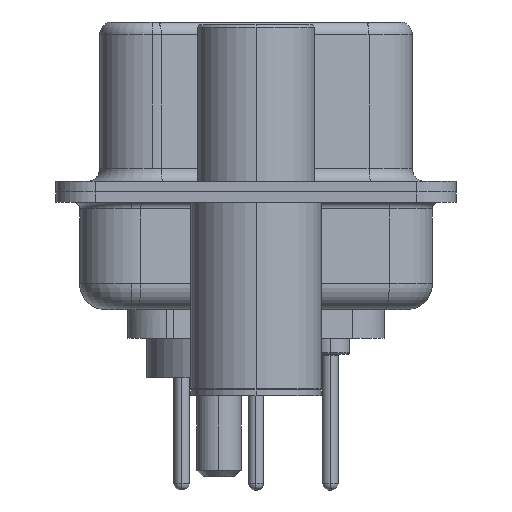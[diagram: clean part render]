
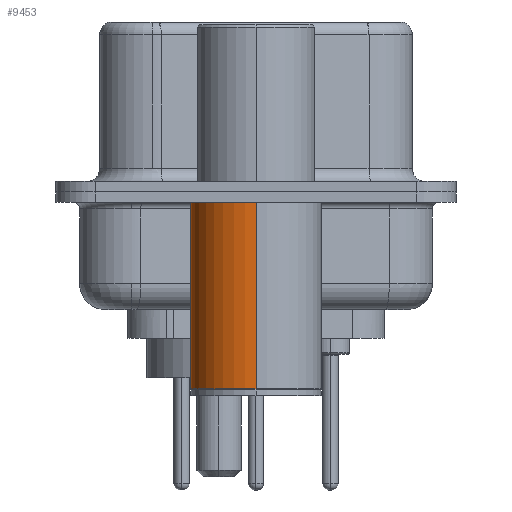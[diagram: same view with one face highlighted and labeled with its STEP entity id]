
A CAD part, left-side view. The second image highlights one B-rep face of the part: STEP entity #9453.
In plain terms, the highlighted cylindrical face has radius 2.5 mm (diameter 5 mm), a partial arc.
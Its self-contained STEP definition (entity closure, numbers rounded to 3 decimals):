
#170 = CYLINDRICAL_SURFACE ( 'NONE', #28979, 2.5 ) ;
#680 = CIRCLE ( 'NONE', #1259, 2.5 ) ;
#879 = ORIENTED_EDGE ( 'NONE', *, *, #28525, .T. ) ;
#1050 = CARTESIAN_POINT ( 'NONE',  ( -2.5, 0., -0.4 ) ) ;
#1259 = AXIS2_PLACEMENT_3D ( 'NONE', #6846, #24895, #9473 ) ;
#1789 = DIRECTION ( 'NONE',  ( 0., 0., 1. ) ) ;
#1864 = DIRECTION ( 'NONE',  ( 0., 0., 1. ) ) ;
#3225 = DIRECTION ( 'NONE',  ( 0., 0., 1. ) ) ;
#3404 = CARTESIAN_POINT ( 'NONE',  ( 2.5, 0., -7.525 ) ) ;
#3531 = FACE_OUTER_BOUND ( 'NONE', #16868, .T. ) ;
#4722 = LINE ( 'NONE', #8339, #30460 ) ;
#4806 = LINE ( 'NONE', #27537, #24554 ) ;
#6846 = CARTESIAN_POINT ( 'NONE',  ( 0., 0., -7.525 ) ) ;
#7082 = DIRECTION ( 'NONE',  ( 1., 0., 0. ) ) ;
#7803 = EDGE_CURVE ( 'NONE', #16763, #17645, #20937, .T. ) ;
#8339 = CARTESIAN_POINT ( 'NONE',  ( 2.5, 0., 0.581 ) ) ;
#9453 = ADVANCED_FACE ( 'NONE', ( #3531 ), #170, .T. ) ;
#9473 = DIRECTION ( 'NONE',  ( 1., 0., 0. ) ) ;
#10934 = DIRECTION ( 'NONE',  ( 0., 0., 1. ) ) ;
#16763 = VERTEX_POINT ( 'NONE', #20075 ) ;
#16868 = EDGE_LOOP ( 'NONE', ( #879, #17960, #17352, #31605 ) ) ;
#17352 = ORIENTED_EDGE ( 'NONE', *, *, #7803, .F. ) ;
#17645 = VERTEX_POINT ( 'NONE', #1050 ) ;
#17960 = ORIENTED_EDGE ( 'NONE', *, *, #31916, .T. ) ;
#18498 = AXIS2_PLACEMENT_3D ( 'NONE', #18704, #3225, #21241 ) ;
#18704 = CARTESIAN_POINT ( 'NONE',  ( 0., 0., -0.4 ) ) ;
#20075 = CARTESIAN_POINT ( 'NONE',  ( 2.5, 0., -0.4 ) ) ;
#20937 = CIRCLE ( 'NONE', #18498, 2.5 ) ;
#21241 = DIRECTION ( 'NONE',  ( 1., 0., 0. ) ) ;
#21891 = EDGE_CURVE ( 'NONE', #30395, #16763, #4722, .T. ) ;
#22501 = CARTESIAN_POINT ( 'NONE',  ( 0., 0., 0.581 ) ) ;
#24554 = VECTOR ( 'NONE', #1789, 1000. ) ;
#24895 = DIRECTION ( 'NONE',  ( 0., 0., 1. ) ) ;
#27537 = CARTESIAN_POINT ( 'NONE',  ( -2.5, 0., 0.581 ) ) ;
#28525 = EDGE_CURVE ( 'NONE', #30395, #31886, #680, .T. ) ;
#28979 = AXIS2_PLACEMENT_3D ( 'NONE', #22501, #1864, #7082 ) ;
#29967 = CARTESIAN_POINT ( 'NONE',  ( -2.5, 0., -7.525 ) ) ;
#30395 = VERTEX_POINT ( 'NONE', #3404 ) ;
#30460 = VECTOR ( 'NONE', #10934, 1000. ) ;
#31605 = ORIENTED_EDGE ( 'NONE', *, *, #21891, .F. ) ;
#31886 = VERTEX_POINT ( 'NONE', #29967 ) ;
#31916 = EDGE_CURVE ( 'NONE', #31886, #17645, #4806, .T. ) ;
